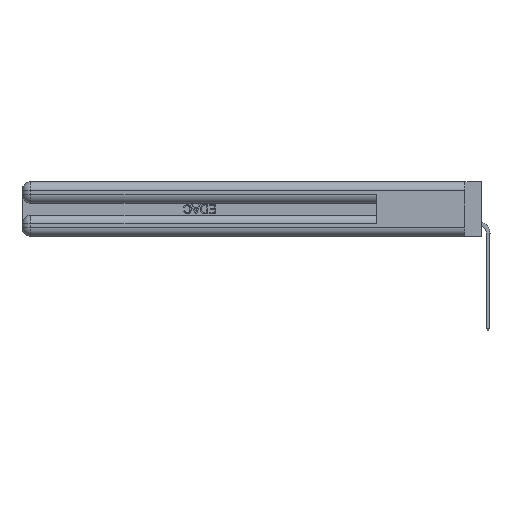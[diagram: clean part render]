
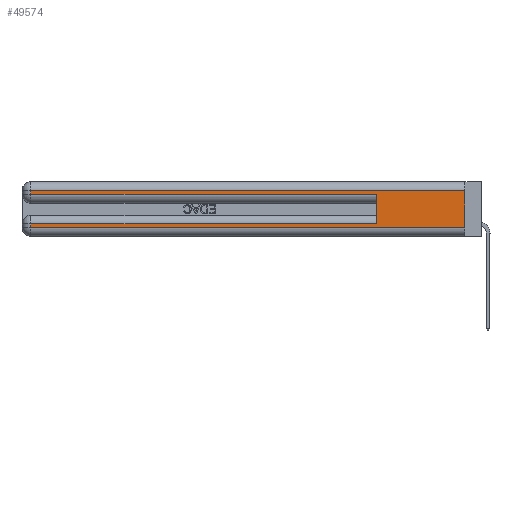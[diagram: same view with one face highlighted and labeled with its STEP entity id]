
A CAD part, left-side view. The second image highlights one B-rep face of the part: STEP entity #49574.
In plain terms, the highlighted planar face has unit normal (-1, 0, 0).
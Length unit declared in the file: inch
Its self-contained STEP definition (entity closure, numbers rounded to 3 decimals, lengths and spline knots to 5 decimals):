
#438 = DIRECTION ( 'NONE',  ( 0., 1., 0. ) ) ;
#4605 = VECTOR ( 'NONE', #38462, 39.37008 ) ;
#4792 = DIRECTION ( 'NONE',  ( 0., 0., -1. ) ) ;
#5137 = DIRECTION ( 'NONE',  ( 0., -1., 0. ) ) ;
#5545 = ORIENTED_EDGE ( 'NONE', *, *, #48257, .T. ) ;
#7262 = LINE ( 'NONE', #43106, #4605 ) ;
#7645 = ORIENTED_EDGE ( 'NONE', *, *, #21536, .T. ) ;
#8758 = DIRECTION ( 'NONE',  ( 0., -1., 0. ) ) ;
#9235 = CARTESIAN_POINT ( 'NONE',  ( 0., 0., 0.37 ) ) ;
#9348 = LINE ( 'NONE', #25186, #19102 ) ;
#9808 = FACE_OUTER_BOUND ( 'NONE', #34419, .T. ) ;
#11947 = LINE ( 'NONE', #42558, #18310 ) ;
#13449 = CARTESIAN_POINT ( 'NONE',  ( 0., 0.6, 0.285 ) ) ;
#13508 = EDGE_CURVE ( 'NONE', #41651, #18863, #7262, .T. ) ;
#13715 = ORIENTED_EDGE ( 'NONE', *, *, #28416, .F. ) ;
#14245 = VECTOR ( 'NONE', #24281, 39.37008 ) ;
#16342 = EDGE_CURVE ( 'NONE', #41055, #17904, #16618, .T. ) ;
#16618 = LINE ( 'NONE', #51116, #41514 ) ;
#17637 = DIRECTION ( 'NONE',  ( 0., 0., 1. ) ) ;
#17904 = VERTEX_POINT ( 'NONE', #36193 ) ;
#18024 = LINE ( 'NONE', #25754, #34712 ) ;
#18310 = VECTOR ( 'NONE', #5137, 39.37008 ) ;
#18359 = EDGE_CURVE ( 'NONE', #17904, #18863, #11947, .T. ) ;
#18863 = VERTEX_POINT ( 'NONE', #38038 ) ;
#19102 = VECTOR ( 'NONE', #19892, 39.37008 ) ;
#19892 = DIRECTION ( 'NONE',  ( 0., 0., -1. ) ) ;
#20224 = VERTEX_POINT ( 'NONE', #13449 ) ;
#20958 = DIRECTION ( 'NONE',  ( 1., 0., 0. ) ) ;
#21428 = VERTEX_POINT ( 'NONE', #23227 ) ;
#21536 = EDGE_CURVE ( 'NONE', #21428, #41055, #51450, .T. ) ;
#21827 = CARTESIAN_POINT ( 'NONE',  ( 0., 2.94, 0.31 ) ) ;
#23227 = CARTESIAN_POINT ( 'NONE',  ( 0., 0.6, 0.085 ) ) ;
#24105 = CARTESIAN_POINT ( 'NONE',  ( 0., 0., 0.085 ) ) ;
#24207 = EDGE_CURVE ( 'NONE', #49318, #46071, #9348, .T. ) ;
#24281 = DIRECTION ( 'NONE',  ( 0., 1., 0. ) ) ;
#25186 = CARTESIAN_POINT ( 'NONE',  ( 0., 2.94, 0.37 ) ) ;
#25617 = ORIENTED_EDGE ( 'NONE', *, *, #13508, .F. ) ;
#25754 = CARTESIAN_POINT ( 'NONE',  ( 0., 0., 0.285 ) ) ;
#28416 = EDGE_CURVE ( 'NONE', #21428, #20224, #41767, .T. ) ;
#29657 = CARTESIAN_POINT ( 'NONE',  ( 0., 0.6, 0.145 ) ) ;
#29862 = LINE ( 'NONE', #45300, #48563 ) ;
#32679 = ORIENTED_EDGE ( 'NONE', *, *, #18359, .T. ) ;
#33469 = ORIENTED_EDGE ( 'NONE', *, *, #16342, .T. ) ;
#34419 = EDGE_LOOP ( 'NONE', ( #25617, #5545, #41957, #41559, #13715, #7645, #33469, #32679 ) ) ;
#34712 = VECTOR ( 'NONE', #8758, 39.37008 ) ;
#36193 = CARTESIAN_POINT ( 'NONE',  ( 0., 2.94, 0.06 ) ) ;
#37231 = CARTESIAN_POINT ( 'NONE',  ( 0., 0., 0.31 ) ) ;
#37705 = AXIS2_PLACEMENT_3D ( 'NONE', #9235, #20958, #4792 ) ;
#38038 = CARTESIAN_POINT ( 'NONE',  ( 0., 0., 0.06 ) ) ;
#38462 = DIRECTION ( 'NONE',  ( 0., 0., -1. ) ) ;
#41055 = VERTEX_POINT ( 'NONE', #50803 ) ;
#41514 = VECTOR ( 'NONE', #46741, 39.37008 ) ;
#41559 = ORIENTED_EDGE ( 'NONE', *, *, #52786, .T. ) ;
#41651 = VERTEX_POINT ( 'NONE', #37231 ) ;
#41767 = LINE ( 'NONE', #29657, #51482 ) ;
#41957 = ORIENTED_EDGE ( 'NONE', *, *, #24207, .T. ) ;
#42558 = CARTESIAN_POINT ( 'NONE',  ( 0., 0., 0.06 ) ) ;
#43106 = CARTESIAN_POINT ( 'NONE',  ( 0., 0., 0.37 ) ) ;
#43391 = CARTESIAN_POINT ( 'NONE',  ( 0., 2.94, 0.285 ) ) ;
#45300 = CARTESIAN_POINT ( 'NONE',  ( 0., 0., 0.31 ) ) ;
#45960 = PLANE ( 'NONE',  #37705 ) ;
#46071 = VERTEX_POINT ( 'NONE', #43391 ) ;
#46741 = DIRECTION ( 'NONE',  ( 0., 0., -1. ) ) ;
#48257 = EDGE_CURVE ( 'NONE', #41651, #49318, #29862, .T. ) ;
#48563 = VECTOR ( 'NONE', #438, 39.37008 ) ;
#49318 = VERTEX_POINT ( 'NONE', #21827 ) ;
#49574 = ADVANCED_FACE ( 'NONE', ( #9808 ), #45960, .F. ) ;
#50803 = CARTESIAN_POINT ( 'NONE',  ( 0., 2.94, 0.085 ) ) ;
#51116 = CARTESIAN_POINT ( 'NONE',  ( 0., 2.94, 0.37 ) ) ;
#51450 = LINE ( 'NONE', #24105, #14245 ) ;
#51482 = VECTOR ( 'NONE', #17637, 39.37008 ) ;
#52786 = EDGE_CURVE ( 'NONE', #46071, #20224, #18024, .T. ) ;
